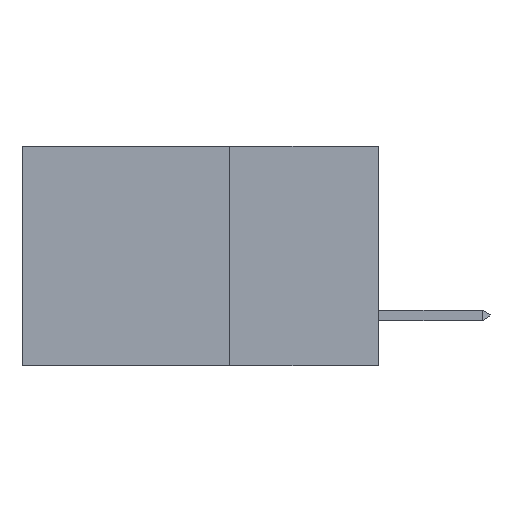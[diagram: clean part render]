
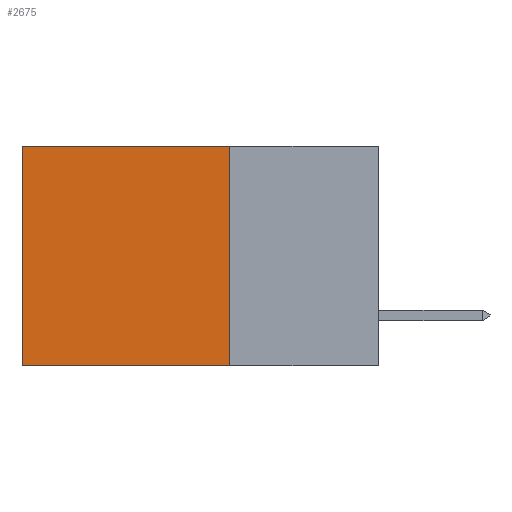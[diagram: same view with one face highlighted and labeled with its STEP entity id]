
A CAD part, left-side view. The second image highlights one B-rep face of the part: STEP entity #2675.
In plain terms, the highlighted planar face has unit normal (-1, 0, 0).
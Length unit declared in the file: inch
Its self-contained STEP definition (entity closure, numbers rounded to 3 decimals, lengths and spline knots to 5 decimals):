
#1002 = DIRECTION ( 'NONE',  ( 1., 0., 0. ) ) ;
#2519 = EDGE_CURVE ( 'NONE', #9788, #14555, #7846, .T. ) ;
#2675 = ADVANCED_FACE ( 'NONE', ( #9127 ), #8012, .F. ) ;
#3085 = AXIS2_PLACEMENT_3D ( 'NONE', #11476, #1002, #4450 ) ;
#3641 = CARTESIAN_POINT ( 'NONE',  ( 0.298, 0.25, 0. ) ) ;
#3693 = CARTESIAN_POINT ( 'NONE',  ( 0.298, 0.25, -0.37 ) ) ;
#3694 = DIRECTION ( 'NONE',  ( 0., 1., 0. ) ) ;
#3747 = CARTESIAN_POINT ( 'NONE',  ( 0.298, 0.6, 0. ) ) ;
#3862 = ORIENTED_EDGE ( 'NONE', *, *, #13181, .F. ) ;
#4315 = EDGE_CURVE ( 'NONE', #12723, #14791, #12177, .T. ) ;
#4357 = VECTOR ( 'NONE', #9749, 39.37008 ) ;
#4450 = DIRECTION ( 'NONE',  ( 0., 0., -1. ) ) ;
#6620 = CARTESIAN_POINT ( 'NONE',  ( 0.298, 0.6, 0. ) ) ;
#6771 = EDGE_CURVE ( 'NONE', #14555, #14791, #13592, .T. ) ;
#7455 = CARTESIAN_POINT ( 'NONE',  ( 0.298, 0.6, -0.37 ) ) ;
#7846 = LINE ( 'NONE', #3641, #8567 ) ;
#7886 = DIRECTION ( 'NONE',  ( 0., 0., -1. ) ) ;
#8012 = PLANE ( 'NONE',  #3085 ) ;
#8567 = VECTOR ( 'NONE', #3694, 39.37008 ) ;
#8715 = ORIENTED_EDGE ( 'NONE', *, *, #4315, .F. ) ;
#9127 = FACE_OUTER_BOUND ( 'NONE', #14059, .T. ) ;
#9749 = DIRECTION ( 'NONE',  ( 0., 1., 0. ) ) ;
#9788 = VERTEX_POINT ( 'NONE', #14933 ) ;
#9804 = CARTESIAN_POINT ( 'NONE',  ( 0.298, 0.25, -0.37 ) ) ;
#10429 = VECTOR ( 'NONE', #7886, 39.37008 ) ;
#11476 = CARTESIAN_POINT ( 'NONE',  ( 0.298, 0.25, 0. ) ) ;
#12177 = LINE ( 'NONE', #9804, #4357 ) ;
#12723 = VERTEX_POINT ( 'NONE', #3693 ) ;
#12752 = CARTESIAN_POINT ( 'NONE',  ( 0.298, 0.25, 0. ) ) ;
#13181 = EDGE_CURVE ( 'NONE', #9788, #12723, #13306, .T. ) ;
#13183 = ORIENTED_EDGE ( 'NONE', *, *, #2519, .T. ) ;
#13306 = LINE ( 'NONE', #12752, #13867 ) ;
#13592 = LINE ( 'NONE', #6620, #10429 ) ;
#13867 = VECTOR ( 'NONE', #15130, 39.37008 ) ;
#14059 = EDGE_LOOP ( 'NONE', ( #14866, #8715, #3862, #13183 ) ) ;
#14555 = VERTEX_POINT ( 'NONE', #3747 ) ;
#14791 = VERTEX_POINT ( 'NONE', #7455 ) ;
#14866 = ORIENTED_EDGE ( 'NONE', *, *, #6771, .T. ) ;
#14933 = CARTESIAN_POINT ( 'NONE',  ( 0.298, 0.25, 0. ) ) ;
#15130 = DIRECTION ( 'NONE',  ( 0., 0., -1. ) ) ;
